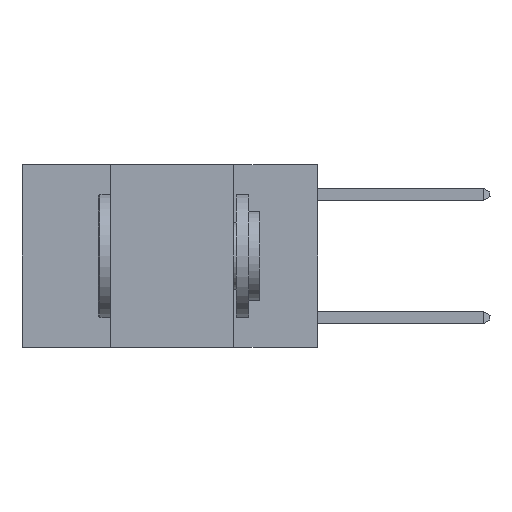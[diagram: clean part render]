
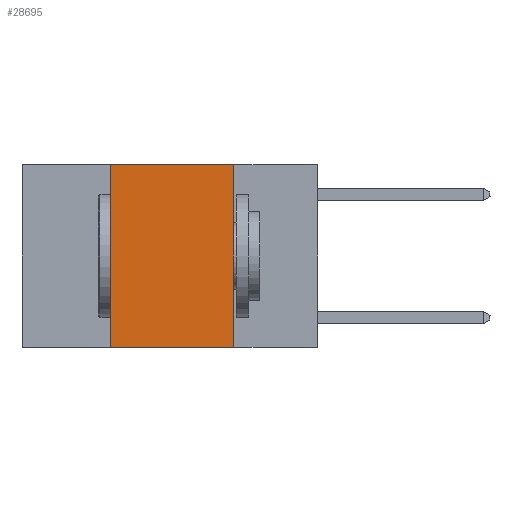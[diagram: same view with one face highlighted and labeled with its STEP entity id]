
A CAD part, left-side view. The second image highlights one B-rep face of the part: STEP entity #28695.
In plain terms, the highlighted planar face has unit normal (-1, 0, 0).
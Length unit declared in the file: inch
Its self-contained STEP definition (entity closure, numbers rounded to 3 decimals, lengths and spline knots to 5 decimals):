
#393 = VECTOR ( 'NONE', #13588, 39.37008 ) ;
#501 = CARTESIAN_POINT ( 'NONE',  ( 0., 0.6, 0. ) ) ;
#1556 = AXIS2_PLACEMENT_3D ( 'NONE', #501, #19908, #5411 ) ;
#2412 = DIRECTION ( 'NONE',  ( 0., 0., 1. ) ) ;
#2944 = PLANE ( 'NONE',  #1556 ) ;
#4290 = CARTESIAN_POINT ( 'NONE',  ( 0., 0.42, -0.37 ) ) ;
#5411 = DIRECTION ( 'NONE',  ( 0., 0., -1. ) ) ;
#6277 = CARTESIAN_POINT ( 'NONE',  ( 0., 0.17, -0.37 ) ) ;
#6340 = CARTESIAN_POINT ( 'NONE',  ( 0., 0.6, -0.37 ) ) ;
#6404 = VECTOR ( 'NONE', #16123, 39.37008 ) ;
#7580 = DIRECTION ( 'NONE',  ( 0., 0., -1. ) ) ;
#7650 = LINE ( 'NONE', #23126, #393 ) ;
#9150 = EDGE_CURVE ( 'NONE', #19517, #9371, #28297, .T. ) ;
#9371 = VERTEX_POINT ( 'NONE', #27245 ) ;
#13588 = DIRECTION ( 'NONE',  ( 0., -1., 0. ) ) ;
#13779 = EDGE_CURVE ( 'NONE', #9371, #18852, #7650, .T. ) ;
#14437 = VECTOR ( 'NONE', #7580, 39.37008 ) ;
#14987 = ORIENTED_EDGE ( 'NONE', *, *, #25592, .F. ) ;
#16123 = DIRECTION ( 'NONE',  ( 0., -1., 0. ) ) ;
#18326 = FACE_OUTER_BOUND ( 'NONE', #19719, .T. ) ;
#18852 = VERTEX_POINT ( 'NONE', #19067 ) ;
#19067 = CARTESIAN_POINT ( 'NONE',  ( 0., 0.17, 0. ) ) ;
#19517 = VERTEX_POINT ( 'NONE', #4290 ) ;
#19719 = EDGE_LOOP ( 'NONE', ( #14987, #20641, #27813, #23612 ) ) ;
#19908 = DIRECTION ( 'NONE',  ( 1., 0., 0. ) ) ;
#20641 = ORIENTED_EDGE ( 'NONE', *, *, #13779, .F. ) ;
#20772 = EDGE_CURVE ( 'NONE', #19517, #22056, #21484, .T. ) ;
#21484 = LINE ( 'NONE', #6340, #6404 ) ;
#21877 = VECTOR ( 'NONE', #2412, 39.37008 ) ;
#22056 = VERTEX_POINT ( 'NONE', #6277 ) ;
#23126 = CARTESIAN_POINT ( 'NONE',  ( 0., 0.6, 0. ) ) ;
#23612 = ORIENTED_EDGE ( 'NONE', *, *, #20772, .T. ) ;
#24061 = CARTESIAN_POINT ( 'NONE',  ( 0., 0.42, 0. ) ) ;
#24343 = CARTESIAN_POINT ( 'NONE',  ( 0., 0.17, 0. ) ) ;
#25592 = EDGE_CURVE ( 'NONE', #18852, #22056, #27998, .T. ) ;
#27245 = CARTESIAN_POINT ( 'NONE',  ( 0., 0.42, 0. ) ) ;
#27813 = ORIENTED_EDGE ( 'NONE', *, *, #9150, .F. ) ;
#27998 = LINE ( 'NONE', #24343, #14437 ) ;
#28297 = LINE ( 'NONE', #24061, #21877 ) ;
#28695 = ADVANCED_FACE ( 'NONE', ( #18326 ), #2944, .F. ) ;
